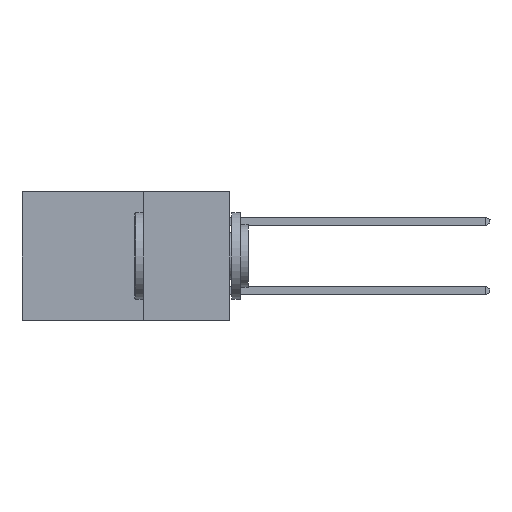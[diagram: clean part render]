
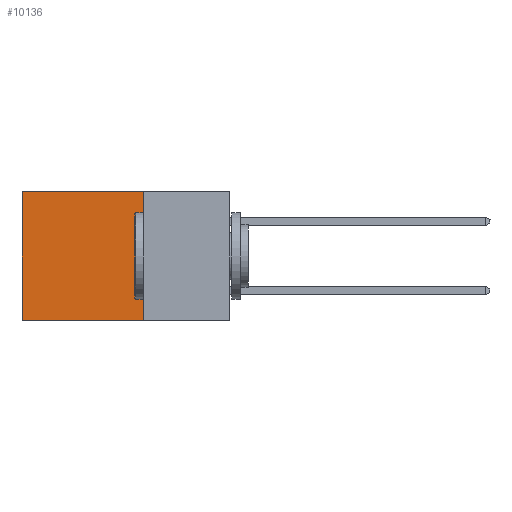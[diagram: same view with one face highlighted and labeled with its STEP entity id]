
A CAD part, left-side view. The second image highlights one B-rep face of the part: STEP entity #10136.
In plain terms, the highlighted planar face has unit normal (-1, 0, 0).
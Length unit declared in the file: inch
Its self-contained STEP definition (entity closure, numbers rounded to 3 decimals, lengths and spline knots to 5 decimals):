
#1108 = ORIENTED_EDGE ( 'NONE', *, *, #9013, .T. ) ;
#1697 = LINE ( 'NONE', #6451, #5728 ) ;
#4006 = VERTEX_POINT ( 'NONE', #7760 ) ;
#4229 = VERTEX_POINT ( 'NONE', #14651 ) ;
#4289 = DIRECTION ( 'NONE',  ( 0., 1., 0. ) ) ;
#4427 = VECTOR ( 'NONE', #12492, 39.37008 ) ;
#4577 = DIRECTION ( 'NONE',  ( 1., 0., 0. ) ) ;
#5055 = LINE ( 'NONE', #8685, #12873 ) ;
#5432 = CARTESIAN_POINT ( 'NONE',  ( 0.2615, 0.25, -0.37 ) ) ;
#5728 = VECTOR ( 'NONE', #12615, 39.37008 ) ;
#5730 = CARTESIAN_POINT ( 'NONE',  ( 0.2615, 0.25, -0.37 ) ) ;
#6059 = ORIENTED_EDGE ( 'NONE', *, *, #12808, .F. ) ;
#6451 = CARTESIAN_POINT ( 'NONE',  ( 0.2615, 0.6, -0.37 ) ) ;
#7708 = EDGE_LOOP ( 'NONE', ( #11903, #6059, #8567, #1108 ) ) ;
#7760 = CARTESIAN_POINT ( 'NONE',  ( 0.2615, 0.25, 0. ) ) ;
#8567 = ORIENTED_EDGE ( 'NONE', *, *, #11184, .F. ) ;
#8685 = CARTESIAN_POINT ( 'NONE',  ( 0.2615, 0.25, -0.37 ) ) ;
#9013 = EDGE_CURVE ( 'NONE', #4006, #12191, #10137, .T. ) ;
#9043 = FACE_OUTER_BOUND ( 'NONE', #7708, .T. ) ;
#10136 = ADVANCED_FACE ( 'NONE', ( #9043 ), #11638, .F. ) ;
#10137 = LINE ( 'NONE', #11162, #4427 ) ;
#11162 = CARTESIAN_POINT ( 'NONE',  ( 0.2615, 0.25, 0. ) ) ;
#11184 = EDGE_CURVE ( 'NONE', #4006, #12238, #5055, .T. ) ;
#11210 = CARTESIAN_POINT ( 'NONE',  ( 0.2615, 0.6, 0. ) ) ;
#11638 = PLANE ( 'NONE',  #14372 ) ;
#11903 = ORIENTED_EDGE ( 'NONE', *, *, #13640, .T. ) ;
#12191 = VERTEX_POINT ( 'NONE', #11210 ) ;
#12238 = VERTEX_POINT ( 'NONE', #14856 ) ;
#12492 = DIRECTION ( 'NONE',  ( 0., 1., 0. ) ) ;
#12615 = DIRECTION ( 'NONE',  ( 0., 0., -1. ) ) ;
#12808 = EDGE_CURVE ( 'NONE', #12238, #4229, #13827, .T. ) ;
#12873 = VECTOR ( 'NONE', #13525, 39.37008 ) ;
#13401 = VECTOR ( 'NONE', #4289, 39.37008 ) ;
#13525 = DIRECTION ( 'NONE',  ( 0., 0., -1. ) ) ;
#13640 = EDGE_CURVE ( 'NONE', #12191, #4229, #1697, .T. ) ;
#13827 = LINE ( 'NONE', #5432, #13401 ) ;
#14351 = DIRECTION ( 'NONE',  ( 0., 0., -1. ) ) ;
#14372 = AXIS2_PLACEMENT_3D ( 'NONE', #5730, #4577, #14351 ) ;
#14651 = CARTESIAN_POINT ( 'NONE',  ( 0.2615, 0.6, -0.37 ) ) ;
#14856 = CARTESIAN_POINT ( 'NONE',  ( 0.2615, 0.25, -0.37 ) ) ;
